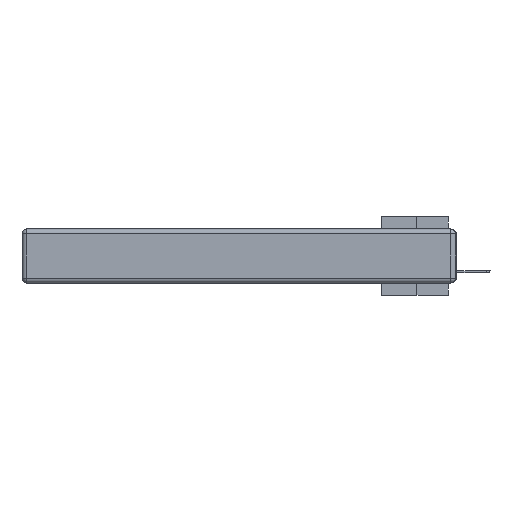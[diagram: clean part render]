
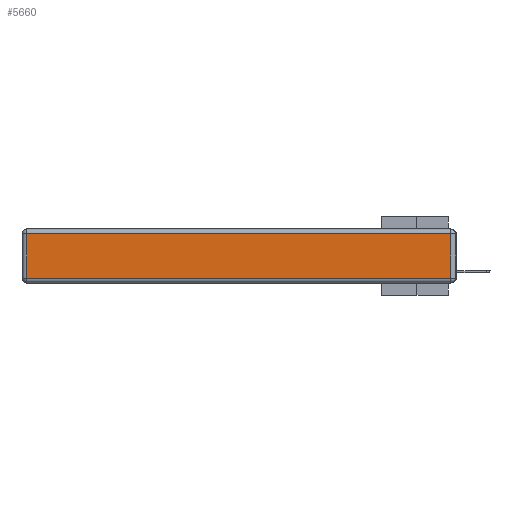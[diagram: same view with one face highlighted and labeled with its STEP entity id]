
A CAD part, left-side view. The second image highlights one B-rep face of the part: STEP entity #5660.
In plain terms, the highlighted planar face has unit normal (-1, 0, 0).
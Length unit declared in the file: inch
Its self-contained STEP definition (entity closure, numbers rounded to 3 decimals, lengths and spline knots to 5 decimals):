
#318 = VECTOR ( 'NONE', #9684, 39.37008 ) ;
#2014 = AXIS2_PLACEMENT_3D ( 'NONE', #9134, #19257, #8798 ) ;
#2623 = CARTESIAN_POINT ( 'NONE',  ( 0., 2.72, -0.03 ) ) ;
#2709 = CARTESIAN_POINT ( 'NONE',  ( 0., 0.03, -0.03 ) ) ;
#2906 = DIRECTION ( 'NONE',  ( 0., 0., 1. ) ) ;
#3508 = CARTESIAN_POINT ( 'NONE',  ( 0., 2.72, -0.313 ) ) ;
#5660 = ADVANCED_FACE ( 'NONE', ( #24401 ), #31391, .T. ) ;
#6720 = VECTOR ( 'NONE', #2906, 39.37008 ) ;
#6821 = DIRECTION ( 'NONE',  ( 0., 0., -1. ) ) ;
#8391 = ORIENTED_EDGE ( 'NONE', *, *, #29279, .T. ) ;
#8798 = DIRECTION ( 'NONE',  ( 0., 0., 1. ) ) ;
#8819 = LINE ( 'NONE', #18944, #16954 ) ;
#9134 = CARTESIAN_POINT ( 'NONE',  ( 0., 0., -0.343 ) ) ;
#9684 = DIRECTION ( 'NONE',  ( 0., -1., 0. ) ) ;
#13034 = ORIENTED_EDGE ( 'NONE', *, *, #30168, .T. ) ;
#15410 = CARTESIAN_POINT ( 'NONE',  ( 0., 0.03, -0.343 ) ) ;
#15849 = ORIENTED_EDGE ( 'NONE', *, *, #30024, .T. ) ;
#16023 = VERTEX_POINT ( 'NONE', #20438 ) ;
#16954 = VECTOR ( 'NONE', #6821, 39.37008 ) ;
#18806 = VERTEX_POINT ( 'NONE', #3508 ) ;
#18944 = CARTESIAN_POINT ( 'NONE',  ( 0., 2.72, -0.343 ) ) ;
#19257 = DIRECTION ( 'NONE',  ( -1., 0., 0. ) ) ;
#20127 = LINE ( 'NONE', #20298, #24793 ) ;
#20298 = CARTESIAN_POINT ( 'NONE',  ( 0., 2.75, -0.03 ) ) ;
#20438 = CARTESIAN_POINT ( 'NONE',  ( 0., 0.03, -0.313 ) ) ;
#22098 = EDGE_LOOP ( 'NONE', ( #15849, #8391, #13034, #29154 ) ) ;
#23408 = EDGE_CURVE ( 'NONE', #23751, #18806, #8819, .T. ) ;
#23751 = VERTEX_POINT ( 'NONE', #2623 ) ;
#24401 = FACE_OUTER_BOUND ( 'NONE', #22098, .T. ) ;
#24793 = VECTOR ( 'NONE', #31229, 39.37008 ) ;
#26171 = LINE ( 'NONE', #15410, #6720 ) ;
#27274 = CARTESIAN_POINT ( 'NONE',  ( 0., 0., -0.313 ) ) ;
#29154 = ORIENTED_EDGE ( 'NONE', *, *, #23408, .T. ) ;
#29279 = EDGE_CURVE ( 'NONE', #16023, #30975, #26171, .T. ) ;
#30024 = EDGE_CURVE ( 'NONE', #18806, #16023, #32428, .T. ) ;
#30168 = EDGE_CURVE ( 'NONE', #30975, #23751, #20127, .T. ) ;
#30975 = VERTEX_POINT ( 'NONE', #2709 ) ;
#31229 = DIRECTION ( 'NONE',  ( 0., 1., 0. ) ) ;
#31391 = PLANE ( 'NONE',  #2014 ) ;
#32428 = LINE ( 'NONE', #27274, #318 ) ;
